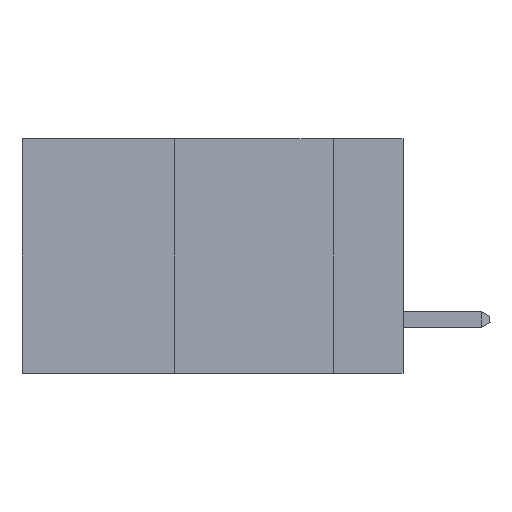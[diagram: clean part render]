
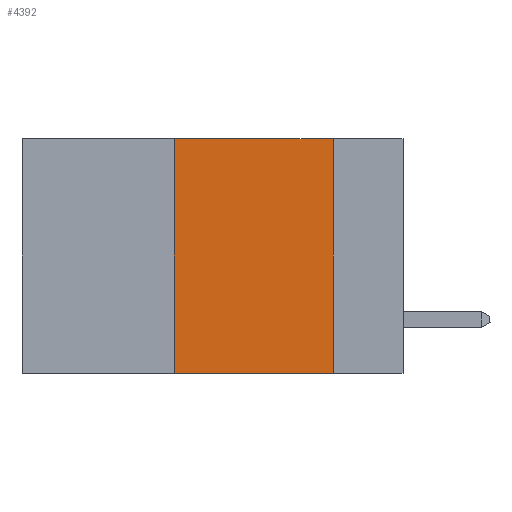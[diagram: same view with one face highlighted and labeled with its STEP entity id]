
A CAD part, left-side view. The second image highlights one B-rep face of the part: STEP entity #4392.
In plain terms, the highlighted planar face has unit normal (-1, 0, 0).
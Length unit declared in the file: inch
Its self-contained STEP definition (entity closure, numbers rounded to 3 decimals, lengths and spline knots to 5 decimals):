
#1721 = CARTESIAN_POINT ( 'NONE',  ( 0., 0.11, 0. ) ) ;
#2631 = CARTESIAN_POINT ( 'NONE',  ( 0., 0.36, 0. ) ) ;
#4392 = ADVANCED_FACE ( 'NONE', ( #18786 ), #32240, .F. ) ;
#4549 = LINE ( 'NONE', #15153, #34176 ) ;
#4590 = CARTESIAN_POINT ( 'NONE',  ( 0., 0.6, 0. ) ) ;
#4973 = AXIS2_PLACEMENT_3D ( 'NONE', #16414, #19678, #19545 ) ;
#5268 = EDGE_CURVE ( 'NONE', #6682, #7206, #18220, .T. ) ;
#5873 = VECTOR ( 'NONE', #15459, 39.37008 ) ;
#6682 = VERTEX_POINT ( 'NONE', #18455 ) ;
#7206 = VERTEX_POINT ( 'NONE', #37751 ) ;
#9857 = ORIENTED_EDGE ( 'NONE', *, *, #14071, .F. ) ;
#10876 = EDGE_CURVE ( 'NONE', #16682, #40777, #13487, .T. ) ;
#11197 = DIRECTION ( 'NONE',  ( 0., -1., 0. ) ) ;
#13327 = ORIENTED_EDGE ( 'NONE', *, *, #10876, .F. ) ;
#13487 = LINE ( 'NONE', #24833, #5873 ) ;
#14071 = EDGE_CURVE ( 'NONE', #7206, #16682, #23456, .T. ) ;
#14555 = EDGE_CURVE ( 'NONE', #6682, #40777, #4549, .T. ) ;
#14990 = DIRECTION ( 'NONE',  ( 0., -1., 0. ) ) ;
#15153 = CARTESIAN_POINT ( 'NONE',  ( 0., 0.6, -0.37 ) ) ;
#15459 = DIRECTION ( 'NONE',  ( 0., 0., -1. ) ) ;
#16414 = CARTESIAN_POINT ( 'NONE',  ( 0., 0.6, 0. ) ) ;
#16682 = VERTEX_POINT ( 'NONE', #1721 ) ;
#17133 = ORIENTED_EDGE ( 'NONE', *, *, #5268, .F. ) ;
#18220 = LINE ( 'NONE', #2631, #25867 ) ;
#18455 = CARTESIAN_POINT ( 'NONE',  ( 0., 0.36, -0.37 ) ) ;
#18786 = FACE_OUTER_BOUND ( 'NONE', #30474, .T. ) ;
#19229 = CARTESIAN_POINT ( 'NONE',  ( 0., 0.11, -0.37 ) ) ;
#19545 = DIRECTION ( 'NONE',  ( 0., 0., -1. ) ) ;
#19678 = DIRECTION ( 'NONE',  ( 1., 0., 0. ) ) ;
#23456 = LINE ( 'NONE', #4590, #33157 ) ;
#24833 = CARTESIAN_POINT ( 'NONE',  ( 0., 0.11, 0. ) ) ;
#25867 = VECTOR ( 'NONE', #32041, 39.37008 ) ;
#30474 = EDGE_LOOP ( 'NONE', ( #13327, #9857, #17133, #31716 ) ) ;
#31716 = ORIENTED_EDGE ( 'NONE', *, *, #14555, .T. ) ;
#32041 = DIRECTION ( 'NONE',  ( 0., 0., 1. ) ) ;
#32240 = PLANE ( 'NONE',  #4973 ) ;
#33157 = VECTOR ( 'NONE', #11197, 39.37008 ) ;
#34176 = VECTOR ( 'NONE', #14990, 39.37008 ) ;
#37751 = CARTESIAN_POINT ( 'NONE',  ( 0., 0.36, 0. ) ) ;
#40777 = VERTEX_POINT ( 'NONE', #19229 ) ;
